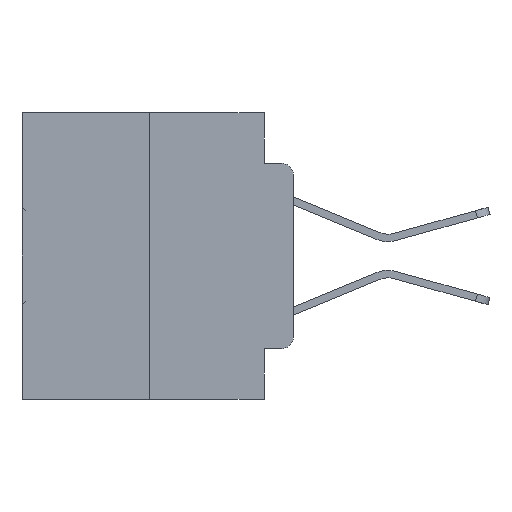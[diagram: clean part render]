
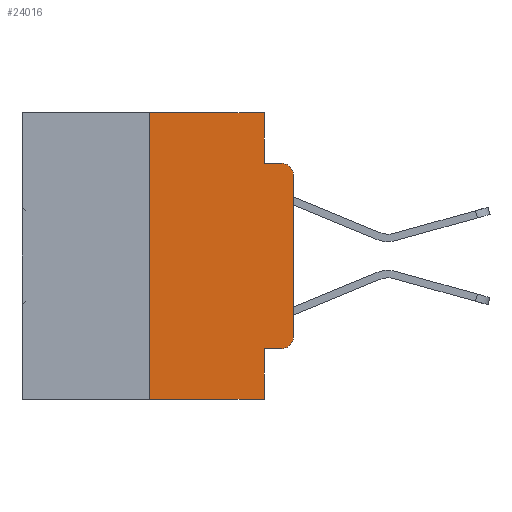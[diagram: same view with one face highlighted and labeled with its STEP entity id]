
A CAD part, left-side view. The second image highlights one B-rep face of the part: STEP entity #24016.
In plain terms, the highlighted planar face has unit normal (-1, 0, 0).
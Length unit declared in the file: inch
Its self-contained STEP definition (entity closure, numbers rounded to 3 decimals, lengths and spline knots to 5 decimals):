
#39 = CARTESIAN_POINT ( 'NONE',  ( 0., 0., -0.3915 ) ) ;
#1189 = DIRECTION ( 'NONE',  ( 0., 0., -1. ) ) ;
#1241 = FACE_OUTER_BOUND ( 'NONE', #12012, .T. ) ;
#1420 = VERTEX_POINT ( 'NONE', #22609 ) ;
#1550 = CARTESIAN_POINT ( 'NONE',  ( 0., 0.02, -0.4115 ) ) ;
#1603 = VECTOR ( 'NONE', #2139, 39.37008 ) ;
#2122 = LINE ( 'NONE', #23124, #2968 ) ;
#2139 = DIRECTION ( 'NONE',  ( 0., 0., -1. ) ) ;
#2250 = EDGE_CURVE ( 'NONE', #12232, #4861, #2122, .T. ) ;
#2404 = CARTESIAN_POINT ( 'NONE',  ( 0., 0.25, 0. ) ) ;
#2739 = DIRECTION ( 'NONE',  ( 0., -1., 0. ) ) ;
#2968 = VECTOR ( 'NONE', #4513, 39.37008 ) ;
#4084 = CARTESIAN_POINT ( 'NONE',  ( 0., 0.473, 0. ) ) ;
#4513 = DIRECTION ( 'NONE',  ( 0., -1., 0. ) ) ;
#4861 = VERTEX_POINT ( 'NONE', #16953 ) ;
#5436 = VECTOR ( 'NONE', #23981, 39.37008 ) ;
#5757 = EDGE_CURVE ( 'NONE', #15529, #23555, #29500, .T. ) ;
#5842 = ORIENTED_EDGE ( 'NONE', *, *, #5757, .T. ) ;
#6295 = PLANE ( 'NONE',  #15968 ) ;
#7077 = CARTESIAN_POINT ( 'NONE',  ( 0., 0.02, -0.3915 ) ) ;
#7336 = ORIENTED_EDGE ( 'NONE', *, *, #26200, .F. ) ;
#7670 = AXIS2_PLACEMENT_3D ( 'NONE', #7077, #25634, #9785 ) ;
#8016 = LINE ( 'NONE', #4084, #21324 ) ;
#8091 = ORIENTED_EDGE ( 'NONE', *, *, #2250, .F. ) ;
#8098 = CARTESIAN_POINT ( 'NONE',  ( 0., 0.473, -0.5 ) ) ;
#8399 = VECTOR ( 'NONE', #2739, 39.37008 ) ;
#8436 = CARTESIAN_POINT ( 'NONE',  ( 0., 0.25, -0.5 ) ) ;
#8698 = VERTEX_POINT ( 'NONE', #8436 ) ;
#9006 = DIRECTION ( 'NONE',  ( 1., 0., 0. ) ) ;
#9363 = CARTESIAN_POINT ( 'NONE',  ( 0., 0.051, 0. ) ) ;
#9785 = DIRECTION ( 'NONE',  ( 0., 0., -1. ) ) ;
#10188 = CIRCLE ( 'NONE', #7670, 0.02 ) ;
#10362 = VERTEX_POINT ( 'NONE', #2404 ) ;
#10396 = ORIENTED_EDGE ( 'NONE', *, *, #25511, .F. ) ;
#10554 = ORIENTED_EDGE ( 'NONE', *, *, #18009, .F. ) ;
#10760 = CARTESIAN_POINT ( 'NONE',  ( 0., 0.02, -0.1085 ) ) ;
#11022 = EDGE_CURVE ( 'NONE', #25140, #12480, #13177, .T. ) ;
#11854 = EDGE_CURVE ( 'NONE', #12480, #4861, #15598, .T. ) ;
#12012 = EDGE_LOOP ( 'NONE', ( #24517, #13260, #8091, #24884, #10554, #7336, #22255, #10396, #5842, #20164 ) ) ;
#12232 = VERTEX_POINT ( 'NONE', #26118 ) ;
#12335 = VECTOR ( 'NONE', #15785, 39.37008 ) ;
#12480 = VERTEX_POINT ( 'NONE', #32183 ) ;
#13083 = EDGE_CURVE ( 'NONE', #8698, #19175, #24985, .T. ) ;
#13177 = LINE ( 'NONE', #28884, #12335 ) ;
#13260 = ORIENTED_EDGE ( 'NONE', *, *, #11854, .T. ) ;
#13464 = DIRECTION ( 'NONE',  ( 0., 0., -1. ) ) ;
#14894 = DIRECTION ( 'NONE',  ( 0., -1., 0. ) ) ;
#15529 = VERTEX_POINT ( 'NONE', #32100 ) ;
#15598 = CIRCLE ( 'NONE', #17457, 0.02 ) ;
#15785 = DIRECTION ( 'NONE',  ( 0., 0., 1. ) ) ;
#15968 = AXIS2_PLACEMENT_3D ( 'NONE', #24865, #9006, #27523 ) ;
#16953 = CARTESIAN_POINT ( 'NONE',  ( 0., 0.02, -0.0885 ) ) ;
#17140 = CARTESIAN_POINT ( 'NONE',  ( 0., 0.051, -0.5 ) ) ;
#17457 = AXIS2_PLACEMENT_3D ( 'NONE', #10760, #29208, #13464 ) ;
#18009 = EDGE_CURVE ( 'NONE', #10362, #1420, #8016, .T. ) ;
#18360 = LINE ( 'NONE', #23571, #31513 ) ;
#18779 = LINE ( 'NONE', #9363, #32759 ) ;
#19175 = VERTEX_POINT ( 'NONE', #17140 ) ;
#20164 = ORIENTED_EDGE ( 'NONE', *, *, #33652, .T. ) ;
#21324 = VECTOR ( 'NONE', #14894, 39.37008 ) ;
#22255 = ORIENTED_EDGE ( 'NONE', *, *, #13083, .T. ) ;
#22609 = CARTESIAN_POINT ( 'NONE',  ( 0., 0.051, 0. ) ) ;
#23124 = CARTESIAN_POINT ( 'NONE',  ( 0., 0.051, -0.0885 ) ) ;
#23555 = VERTEX_POINT ( 'NONE', #1550 ) ;
#23571 = CARTESIAN_POINT ( 'NONE',  ( 0., 0.25, 0. ) ) ;
#23981 = DIRECTION ( 'NONE',  ( 0., -1., 0. ) ) ;
#24016 = ADVANCED_FACE ( 'NONE', ( #1241 ), #6295, .F. ) ;
#24517 = ORIENTED_EDGE ( 'NONE', *, *, #11022, .T. ) ;
#24865 = CARTESIAN_POINT ( 'NONE',  ( 0., 0.473, 0. ) ) ;
#24884 = ORIENTED_EDGE ( 'NONE', *, *, #25953, .F. ) ;
#24985 = LINE ( 'NONE', #8098, #5436 ) ;
#25140 = VERTEX_POINT ( 'NONE', #39 ) ;
#25511 = EDGE_CURVE ( 'NONE', #15529, #19175, #33585, .T. ) ;
#25634 = DIRECTION ( 'NONE',  ( -1., 0., 0. ) ) ;
#25953 = EDGE_CURVE ( 'NONE', #1420, #12232, #18779, .T. ) ;
#26118 = CARTESIAN_POINT ( 'NONE',  ( 0., 0.051, -0.0885 ) ) ;
#26200 = EDGE_CURVE ( 'NONE', #8698, #10362, #18360, .T. ) ;
#26227 = DIRECTION ( 'NONE',  ( 0., 0., 1. ) ) ;
#27523 = DIRECTION ( 'NONE',  ( 0., 0., -1. ) ) ;
#28884 = CARTESIAN_POINT ( 'NONE',  ( 0., 0., 0. ) ) ;
#29208 = DIRECTION ( 'NONE',  ( -1., 0., 0. ) ) ;
#29500 = LINE ( 'NONE', #31916, #8399 ) ;
#31513 = VECTOR ( 'NONE', #26227, 39.37008 ) ;
#31916 = CARTESIAN_POINT ( 'NONE',  ( 0., 0.051, -0.4115 ) ) ;
#32100 = CARTESIAN_POINT ( 'NONE',  ( 0., 0.051, -0.4115 ) ) ;
#32183 = CARTESIAN_POINT ( 'NONE',  ( 0., 0., -0.1085 ) ) ;
#32759 = VECTOR ( 'NONE', #1189, 39.37008 ) ;
#33585 = LINE ( 'NONE', #33920, #1603 ) ;
#33652 = EDGE_CURVE ( 'NONE', #23555, #25140, #10188, .T. ) ;
#33920 = CARTESIAN_POINT ( 'NONE',  ( 0., 0.051, 0. ) ) ;
